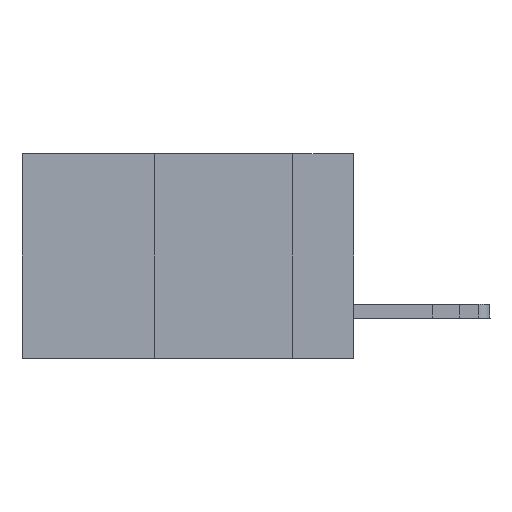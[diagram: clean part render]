
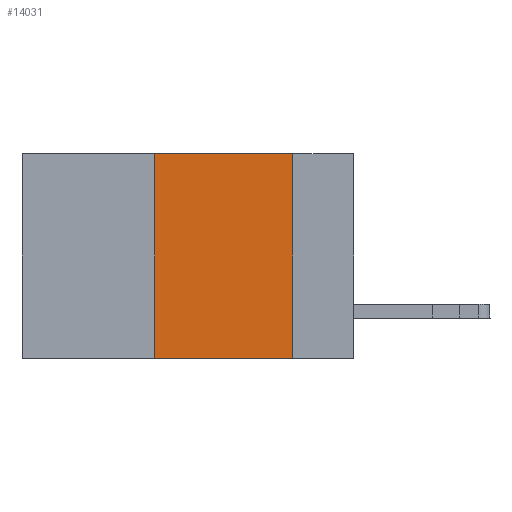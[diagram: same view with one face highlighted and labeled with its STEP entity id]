
A CAD part, left-side view. The second image highlights one B-rep face of the part: STEP entity #14031.
In plain terms, the highlighted planar face has unit normal (-1, 0, 0).
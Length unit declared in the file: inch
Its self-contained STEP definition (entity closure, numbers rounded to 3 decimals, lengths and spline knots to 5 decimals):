
#457 = LINE ( 'NONE', #7775, #19931 ) ;
#2539 = DIRECTION ( 'NONE',  ( 0., -1., 0. ) ) ;
#2779 = DIRECTION ( 'NONE',  ( 0., 0., 1. ) ) ;
#3324 = CARTESIAN_POINT ( 'NONE',  ( 0., 0.11, 0. ) ) ;
#5780 = VERTEX_POINT ( 'NONE', #6105 ) ;
#6105 = CARTESIAN_POINT ( 'NONE',  ( 0., 0.36, 0. ) ) ;
#7277 = CARTESIAN_POINT ( 'NONE',  ( 0., 0.6, -0.37 ) ) ;
#7449 = LINE ( 'NONE', #23641, #19703 ) ;
#7775 = CARTESIAN_POINT ( 'NONE',  ( 0., 0.11, 0. ) ) ;
#7899 = VERTEX_POINT ( 'NONE', #3324 ) ;
#9203 = DIRECTION ( 'NONE',  ( 0., 0., -1. ) ) ;
#9495 = PLANE ( 'NONE',  #15914 ) ;
#10008 = DIRECTION ( 'NONE',  ( 0., 0., -1. ) ) ;
#10189 = FACE_OUTER_BOUND ( 'NONE', #21514, .T. ) ;
#11906 = EDGE_CURVE ( 'NONE', #7899, #14150, #457, .T. ) ;
#12147 = ORIENTED_EDGE ( 'NONE', *, *, #11906, .F. ) ;
#12791 = VECTOR ( 'NONE', #22109, 39.37008 ) ;
#13895 = ORIENTED_EDGE ( 'NONE', *, *, #24016, .T. ) ;
#13955 = EDGE_CURVE ( 'NONE', #5780, #7899, #14191, .T. ) ;
#14031 = ADVANCED_FACE ( 'NONE', ( #10189 ), #9495, .F. ) ;
#14150 = VERTEX_POINT ( 'NONE', #17675 ) ;
#14191 = LINE ( 'NONE', #23853, #18507 ) ;
#14472 = ORIENTED_EDGE ( 'NONE', *, *, #13955, .F. ) ;
#15475 = EDGE_CURVE ( 'NONE', #23878, #5780, #7449, .T. ) ;
#15710 = CARTESIAN_POINT ( 'NONE',  ( 0., 0.6, 0. ) ) ;
#15914 = AXIS2_PLACEMENT_3D ( 'NONE', #15710, #20141, #9203 ) ;
#17675 = CARTESIAN_POINT ( 'NONE',  ( 0., 0.11, -0.37 ) ) ;
#18507 = VECTOR ( 'NONE', #2539, 39.37008 ) ;
#19703 = VECTOR ( 'NONE', #2779, 39.37008 ) ;
#19931 = VECTOR ( 'NONE', #10008, 39.37008 ) ;
#20141 = DIRECTION ( 'NONE',  ( 1., 0., 0. ) ) ;
#20345 = CARTESIAN_POINT ( 'NONE',  ( 0., 0.36, -0.37 ) ) ;
#21514 = EDGE_LOOP ( 'NONE', ( #12147, #14472, #23438, #13895 ) ) ;
#22109 = DIRECTION ( 'NONE',  ( 0., -1., 0. ) ) ;
#23093 = LINE ( 'NONE', #7277, #12791 ) ;
#23438 = ORIENTED_EDGE ( 'NONE', *, *, #15475, .F. ) ;
#23641 = CARTESIAN_POINT ( 'NONE',  ( 0., 0.36, 0. ) ) ;
#23853 = CARTESIAN_POINT ( 'NONE',  ( 0., 0.6, 0. ) ) ;
#23878 = VERTEX_POINT ( 'NONE', #20345 ) ;
#24016 = EDGE_CURVE ( 'NONE', #23878, #14150, #23093, .T. ) ;
